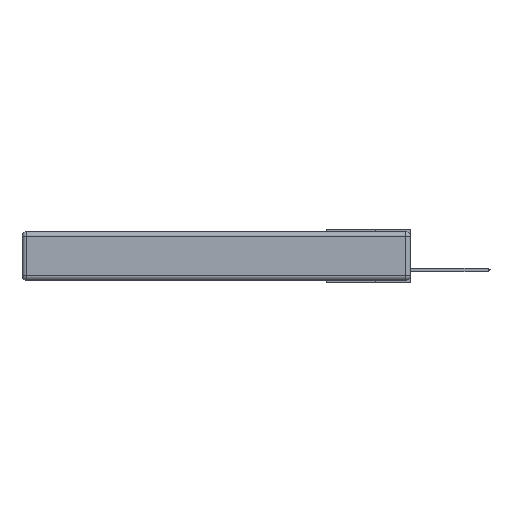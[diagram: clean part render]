
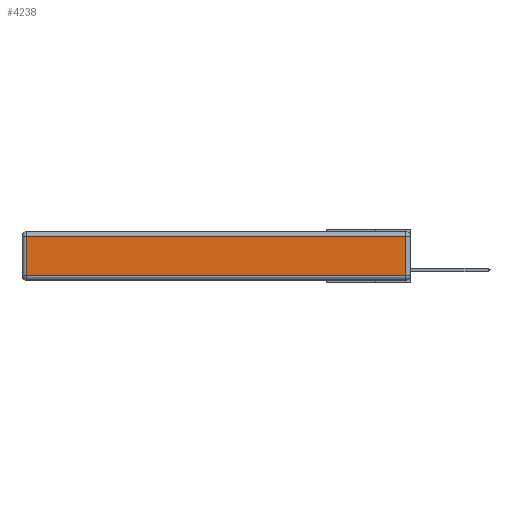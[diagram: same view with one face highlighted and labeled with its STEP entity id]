
A CAD part, left-side view. The second image highlights one B-rep face of the part: STEP entity #4238.
In plain terms, the highlighted planar face has unit normal (-1, 0, 0).
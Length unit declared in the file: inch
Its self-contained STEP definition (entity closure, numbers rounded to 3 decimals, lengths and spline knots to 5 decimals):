
#86 = DIRECTION ( 'NONE',  ( 0., 0., 1. ) ) ;
#170 = ORIENTED_EDGE ( 'NONE', *, *, #11145, .T. ) ;
#203 = PLANE ( 'NONE',  #1095 ) ;
#960 = FACE_OUTER_BOUND ( 'NONE', #3464, .T. ) ;
#1095 = AXIS2_PLACEMENT_3D ( 'NONE', #7168, #8190, #86 ) ;
#1319 = LINE ( 'NONE', #7034, #3555 ) ;
#1376 = ORIENTED_EDGE ( 'NONE', *, *, #10375, .T. ) ;
#1425 = CARTESIAN_POINT ( 'NONE',  ( 0., 2.72, -0.313 ) ) ;
#2994 = DIRECTION ( 'NONE',  ( 0., -1., 0. ) ) ;
#3464 = EDGE_LOOP ( 'NONE', ( #170, #8574, #1376, #6429 ) ) ;
#3544 = VECTOR ( 'NONE', #11149, 39.37008 ) ;
#3555 = VECTOR ( 'NONE', #2994, 39.37008 ) ;
#4238 = ADVANCED_FACE ( 'NONE', ( #960 ), #203, .T. ) ;
#5106 = EDGE_CURVE ( 'NONE', #8992, #12414, #5499, .T. ) ;
#5320 = CARTESIAN_POINT ( 'NONE',  ( 0., 2.72, -0.03 ) ) ;
#5499 = LINE ( 'NONE', #11271, #6780 ) ;
#6429 = ORIENTED_EDGE ( 'NONE', *, *, #5106, .T. ) ;
#6554 = EDGE_CURVE ( 'NONE', #12381, #8095, #11087, .T. ) ;
#6780 = VECTOR ( 'NONE', #9159, 39.37008 ) ;
#6982 = CARTESIAN_POINT ( 'NONE',  ( 0., 0.03, -0.343 ) ) ;
#7034 = CARTESIAN_POINT ( 'NONE',  ( 0., 0., -0.313 ) ) ;
#7168 = CARTESIAN_POINT ( 'NONE',  ( 0., 0., -0.343 ) ) ;
#7965 = CARTESIAN_POINT ( 'NONE',  ( 0., 0.03, -0.313 ) ) ;
#8095 = VERTEX_POINT ( 'NONE', #8335 ) ;
#8190 = DIRECTION ( 'NONE',  ( -1., 0., 0. ) ) ;
#8335 = CARTESIAN_POINT ( 'NONE',  ( 0., 0.03, -0.03 ) ) ;
#8574 = ORIENTED_EDGE ( 'NONE', *, *, #6554, .T. ) ;
#8992 = VERTEX_POINT ( 'NONE', #5320 ) ;
#9159 = DIRECTION ( 'NONE',  ( 0., 0., -1. ) ) ;
#10056 = CARTESIAN_POINT ( 'NONE',  ( 0., 2.75, -0.03 ) ) ;
#10375 = EDGE_CURVE ( 'NONE', #8095, #8992, #11065, .T. ) ;
#11065 = LINE ( 'NONE', #10056, #3544 ) ;
#11087 = LINE ( 'NONE', #6982, #12468 ) ;
#11145 = EDGE_CURVE ( 'NONE', #12414, #12381, #1319, .T. ) ;
#11149 = DIRECTION ( 'NONE',  ( 0., 1., 0. ) ) ;
#11271 = CARTESIAN_POINT ( 'NONE',  ( 0., 2.72, -0.343 ) ) ;
#12381 = VERTEX_POINT ( 'NONE', #7965 ) ;
#12414 = VERTEX_POINT ( 'NONE', #1425 ) ;
#12468 = VECTOR ( 'NONE', #13080, 39.37008 ) ;
#13080 = DIRECTION ( 'NONE',  ( 0., 0., 1. ) ) ;
